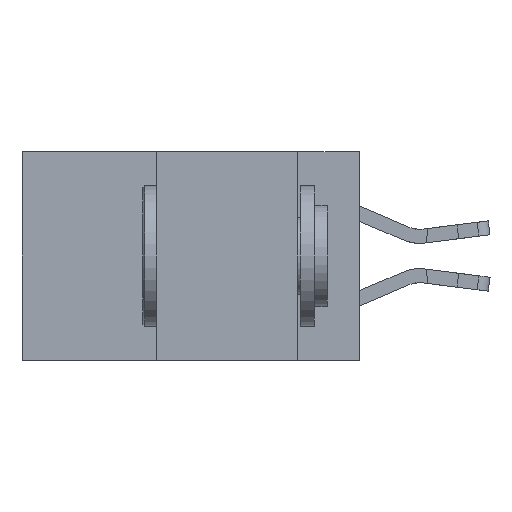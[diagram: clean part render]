
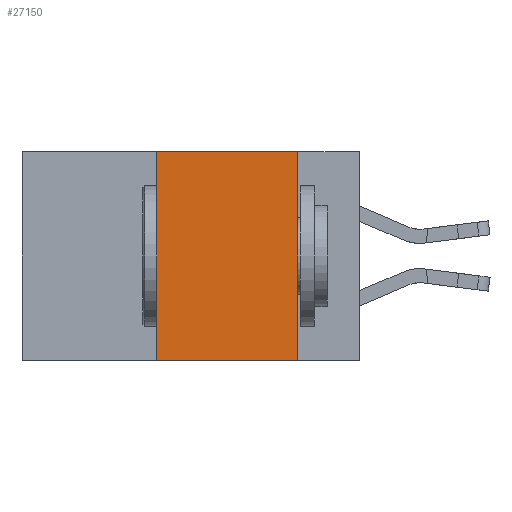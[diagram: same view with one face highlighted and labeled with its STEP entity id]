
A CAD part, left-side view. The second image highlights one B-rep face of the part: STEP entity #27150.
In plain terms, the highlighted planar face has unit normal (-1, 0, 0).
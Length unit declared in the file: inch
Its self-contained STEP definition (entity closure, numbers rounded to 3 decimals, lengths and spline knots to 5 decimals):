
#1455 = CARTESIAN_POINT ( 'NONE',  ( 0., 0.11, -0.37 ) ) ;
#2696 = ORIENTED_EDGE ( 'NONE', *, *, #4478, .F. ) ;
#4031 = CARTESIAN_POINT ( 'NONE',  ( 0., 0.36, 0. ) ) ;
#4153 = DIRECTION ( 'NONE',  ( 1., 0., 0. ) ) ;
#4287 = LINE ( 'NONE', #29529, #8954 ) ;
#4478 = EDGE_CURVE ( 'NONE', #15959, #29178, #29127, .T. ) ;
#5226 = ORIENTED_EDGE ( 'NONE', *, *, #13965, .F. ) ;
#5722 = VECTOR ( 'NONE', #20227, 39.37008 ) ;
#5911 = CARTESIAN_POINT ( 'NONE',  ( 0., 0.36, -0.37 ) ) ;
#6662 = ORIENTED_EDGE ( 'NONE', *, *, #16881, .F. ) ;
#7230 = VECTOR ( 'NONE', #16841, 39.37008 ) ;
#7474 = VERTEX_POINT ( 'NONE', #18640 ) ;
#8954 = VECTOR ( 'NONE', #13773, 39.37008 ) ;
#9872 = EDGE_LOOP ( 'NONE', ( #5226, #6662, #2696, #12439 ) ) ;
#12343 = CARTESIAN_POINT ( 'NONE',  ( 0., 0.11, 0. ) ) ;
#12439 = ORIENTED_EDGE ( 'NONE', *, *, #29062, .T. ) ;
#13687 = VERTEX_POINT ( 'NONE', #1455 ) ;
#13773 = DIRECTION ( 'NONE',  ( 0., -1., 0. ) ) ;
#13965 = EDGE_CURVE ( 'NONE', #7474, #13687, #19256, .T. ) ;
#15738 = CARTESIAN_POINT ( 'NONE',  ( 0., 0.36, 0. ) ) ;
#15959 = VERTEX_POINT ( 'NONE', #5911 ) ;
#16841 = DIRECTION ( 'NONE',  ( 0., 0., -1. ) ) ;
#16881 = EDGE_CURVE ( 'NONE', #29178, #7474, #4287, .T. ) ;
#17074 = VECTOR ( 'NONE', #28569, 39.37008 ) ;
#17781 = CARTESIAN_POINT ( 'NONE',  ( 0., 0.6, 0. ) ) ;
#18640 = CARTESIAN_POINT ( 'NONE',  ( 0., 0.11, 0. ) ) ;
#18758 = AXIS2_PLACEMENT_3D ( 'NONE', #17781, #4153, #20029 ) ;
#19256 = LINE ( 'NONE', #12343, #7230 ) ;
#20029 = DIRECTION ( 'NONE',  ( 0., 0., -1. ) ) ;
#20227 = DIRECTION ( 'NONE',  ( 0., 0., 1. ) ) ;
#21173 = FACE_OUTER_BOUND ( 'NONE', #9872, .T. ) ;
#24024 = CARTESIAN_POINT ( 'NONE',  ( 0., 0.6, -0.37 ) ) ;
#26779 = PLANE ( 'NONE',  #18758 ) ;
#27150 = ADVANCED_FACE ( 'NONE', ( #21173 ), #26779, .F. ) ;
#28569 = DIRECTION ( 'NONE',  ( 0., -1., 0. ) ) ;
#29062 = EDGE_CURVE ( 'NONE', #15959, #13687, #29113, .T. ) ;
#29113 = LINE ( 'NONE', #24024, #17074 ) ;
#29127 = LINE ( 'NONE', #15738, #5722 ) ;
#29178 = VERTEX_POINT ( 'NONE', #4031 ) ;
#29529 = CARTESIAN_POINT ( 'NONE',  ( 0., 0.6, 0. ) ) ;
